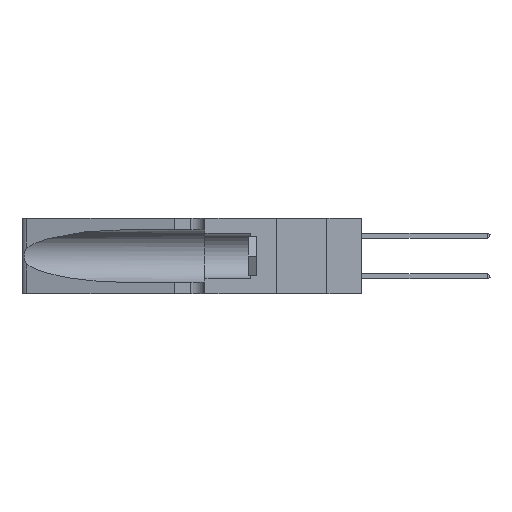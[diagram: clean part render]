
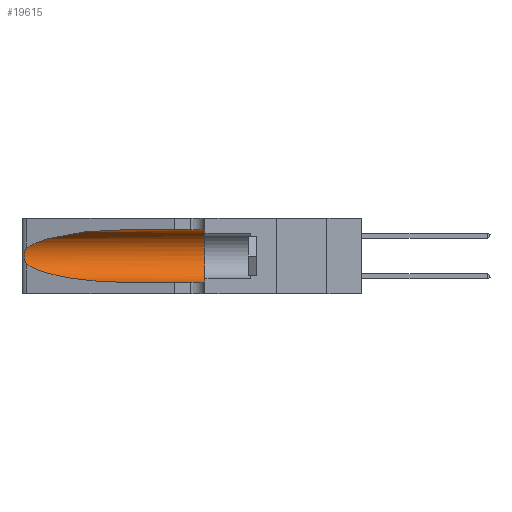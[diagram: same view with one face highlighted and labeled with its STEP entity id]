
A CAD part, left-side view. The second image highlights one B-rep face of the part: STEP entity #19615.
In plain terms, the highlighted cylindrical face has radius 3.308 mm (diameter 6.617 mm), a partial arc.
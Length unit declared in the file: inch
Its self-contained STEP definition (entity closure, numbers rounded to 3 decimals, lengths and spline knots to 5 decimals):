
#432 = DIRECTION ( 'NONE',  ( 0., 1., 0. ) ) ;
#702 = ORIENTED_EDGE ( 'NONE', *, *, #2137, .T. ) ;
#1585 = EDGE_CURVE ( 'NONE', #12105, #1905, #24476, .T. ) ;
#1905 = VERTEX_POINT ( 'NONE', #12191 ) ;
#2059 = CARTESIAN_POINT ( 'NONE',  ( 0.26075, 1.23896, 0.19203 ) ) ;
#2137 = EDGE_CURVE ( 'NONE', #5205, #18317, #16349, .T. ) ;
#2377 = EDGE_CURVE ( 'NONE', #13644, #18317, #21819, .T. ) ;
#2457 = ORIENTED_EDGE ( 'NONE', *, *, #10749, .T. ) ;
#3656 = CARTESIAN_POINT ( 'NONE',  ( 0.1305, 0.72297, 0.31525 ) ) ;
#3894 = CARTESIAN_POINT ( 'NONE',  ( 0.1305, 0.35, 0.05475 ) ) ;
#4334 = CARTESIAN_POINT ( 'NONE',  ( 0.26017, 1.23833, 0.17102 ) ) ;
#5040 = CARTESIAN_POINT ( 'NONE',  ( 0.1305, 1.61858, 0.185 ) ) ;
#5205 = VERTEX_POINT ( 'NONE', #28609 ) ;
#5509 = DIRECTION ( 'NONE',  ( 0., -1., 0. ) ) ;
#5974 = VERTEX_POINT ( 'NONE', #18287 ) ;
#6622 = CARTESIAN_POINT ( 'NONE',  ( 0.25789, 1.23486, 0.15765 ) ) ;
#7686 = AXIS2_PLACEMENT_3D ( 'NONE', #5040, #20667, #25074 ) ;
#7718 = CARTESIAN_POINT ( 'NONE',  ( 0.1305, 1.61858, 0.31525 ) ) ;
#8216 = CARTESIAN_POINT ( 'NONE',  ( 0.25487, 1.22718, 0.22369 ) ) ;
#8885 = CARTESIAN_POINT ( 'NONE',  ( 0.25555, 1.22993, 0.14849 ) ) ;
#8996 =( BOUNDED_CURVE ( )  B_SPLINE_CURVE ( 3, ( #3656, #17119, #21528, #8216 ),
 .UNSPECIFIED., .F., .T. ) 
 B_SPLINE_CURVE_WITH_KNOTS ( ( 4, 4 ),
 ( 1.5708, 2.84003 ),
 .UNSPECIFIED. ) 
 CURVE ( )  GEOMETRIC_REPRESENTATION_ITEM ( )  RATIONAL_B_SPLINE_CURVE ( ( 1., 0.87, 0.87, 1. ) ) 
 REPRESENTATION_ITEM ( '' )  );
#9658 = CARTESIAN_POINT ( 'NONE',  ( 0.25487, 1.22718, 0.14631 ) ) ;
#10749 = EDGE_CURVE ( 'NONE', #5974, #12105, #8996, .T. ) ;
#11033 = CARTESIAN_POINT ( 'NONE',  ( 0.25555, 1.22994, 0.2215 ) ) ;
#11289 = ORIENTED_EDGE ( 'NONE', *, *, #13464, .T. ) ;
#11630 = VECTOR ( 'NONE', #5509, 39.37008 ) ;
#12105 = VERTEX_POINT ( 'NONE', #15396 ) ;
#12191 = CARTESIAN_POINT ( 'NONE',  ( 0.25487, 1.22718, 0.14631 ) ) ;
#13288 = CARTESIAN_POINT ( 'NONE',  ( 0.25787, 1.23484, 0.2124 ) ) ;
#13464 = EDGE_CURVE ( 'NONE', #1905, #5205, #22366, .T. ) ;
#13644 = VERTEX_POINT ( 'NONE', #14755 ) ;
#13925 = CARTESIAN_POINT ( 'NONE',  ( 0.1305, 0.35, 0.185 ) ) ;
#14164 = CARTESIAN_POINT ( 'NONE',  ( 0.1305, 0.72297, 0.05475 ) ) ;
#14755 = CARTESIAN_POINT ( 'NONE',  ( 0.1305, 0.35, 0.31525 ) ) ;
#15122 = AXIS2_PLACEMENT_3D ( 'NONE', #13925, #432, #16203 ) ;
#15396 = CARTESIAN_POINT ( 'NONE',  ( 0.25487, 1.22718, 0.22369 ) ) ;
#15555 = CARTESIAN_POINT ( 'NONE',  ( 0.26018, 1.23835, 0.19895 ) ) ;
#16203 = DIRECTION ( 'NONE',  ( 0., 0., 1. ) ) ;
#16292 = EDGE_LOOP ( 'NONE', ( #2457, #21017, #11289, #702, #26479, #27849 ) ) ;
#16349 = LINE ( 'NONE', #28528, #22186 ) ;
#17119 = CARTESIAN_POINT ( 'NONE',  ( 0.18966, 0.96281, 0.31525 ) ) ;
#17518 = FACE_OUTER_BOUND ( 'NONE', #16292, .T. ) ;
#17776 = CARTESIAN_POINT ( 'NONE',  ( 0.26075, 1.23896, 0.178 ) ) ;
#18287 = CARTESIAN_POINT ( 'NONE',  ( 0.1305, 0.72297, 0.31525 ) ) ;
#18317 = VERTEX_POINT ( 'NONE', #3894 ) ;
#19615 = ADVANCED_FACE ( 'NONE', ( #17518 ), #22679, .F. ) ;
#19880 = CARTESIAN_POINT ( 'NONE',  ( 0.25639, 1.23184, 0.21858 ) ) ;
#19972 = CARTESIAN_POINT ( 'NONE',  ( 0.25856, 1.23593, 0.16098 ) ) ;
#20667 = DIRECTION ( 'NONE',  ( 0., -1., 0. ) ) ;
#21017 = ORIENTED_EDGE ( 'NONE', *, *, #1585, .T. ) ;
#21528 = CARTESIAN_POINT ( 'NONE',  ( 0.2373, 1.15595, 0.28018 ) ) ;
#21819 = CIRCLE ( 'NONE', #15122, 0.13025 ) ;
#22186 = VECTOR ( 'NONE', #24180, 39.37008 ) ;
#22195 = CARTESIAN_POINT ( 'NONE',  ( 0.25639, 1.23186, 0.15144 ) ) ;
#22366 =( BOUNDED_CURVE ( )  B_SPLINE_CURVE ( 3, ( #9658, #22957, #27319, #14164 ),
 .UNSPECIFIED., .F., .T. ) 
 B_SPLINE_CURVE_WITH_KNOTS ( ( 4, 4 ),
 ( 3.44316, 4.71239 ),
 .UNSPECIFIED. ) 
 CURVE ( )  GEOMETRIC_REPRESENTATION_ITEM ( )  RATIONAL_B_SPLINE_CURVE ( ( 1., 0.87, 0.87, 1. ) ) 
 REPRESENTATION_ITEM ( '' )  );
#22679 = CYLINDRICAL_SURFACE ( 'NONE', #7686, 0.13025 ) ;
#22957 = CARTESIAN_POINT ( 'NONE',  ( 0.2373, 1.15595, 0.08982 ) ) ;
#23094 = EDGE_CURVE ( 'NONE', #5974, #13644, #28501, .T. ) ;
#24180 = DIRECTION ( 'NONE',  ( 0., -1., 0. ) ) ;
#24400 = CARTESIAN_POINT ( 'NONE',  ( 0.25487, 1.22718, 0.14631 ) ) ;
#24476 = B_SPLINE_CURVE_WITH_KNOTS ( 'NONE', 3,
 ( #26474, #11033, #19880, #13288, #28657, #15555, #2059, #17776, #4334, #19972, #6622, #22195, #8885, #24400 ),
 .UNSPECIFIED., .F., .F.,
 ( 4, 2, 2, 2, 2, 2, 4 ),
 ( 0., 0.00027, 0.00053, 0.00107, 0.0016, 0.00187, 0.00214 ),
 .UNSPECIFIED. ) ;
#25074 = DIRECTION ( 'NONE',  ( 0., 0., -1. ) ) ;
#26474 = CARTESIAN_POINT ( 'NONE',  ( 0.25487, 1.22718, 0.22369 ) ) ;
#26479 = ORIENTED_EDGE ( 'NONE', *, *, #2377, .F. ) ;
#27319 = CARTESIAN_POINT ( 'NONE',  ( 0.18966, 0.96281, 0.05475 ) ) ;
#27849 = ORIENTED_EDGE ( 'NONE', *, *, #23094, .F. ) ;
#28501 = LINE ( 'NONE', #7718, #11630 ) ;
#28528 = CARTESIAN_POINT ( 'NONE',  ( 0.1305, 1.61858, 0.05475 ) ) ;
#28609 = CARTESIAN_POINT ( 'NONE',  ( 0.1305, 0.72297, 0.05475 ) ) ;
#28657 = CARTESIAN_POINT ( 'NONE',  ( 0.25854, 1.2359, 0.20912 ) ) ;
